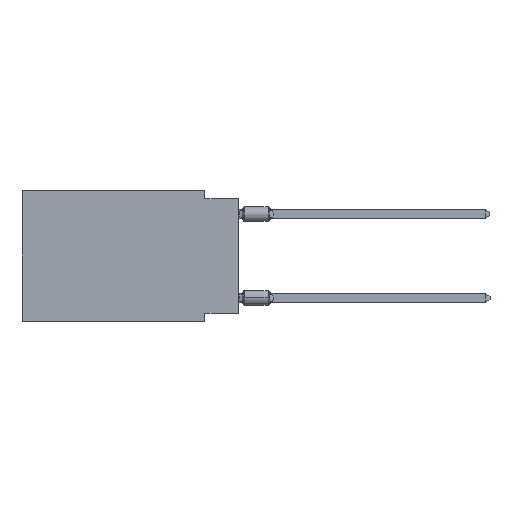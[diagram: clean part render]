
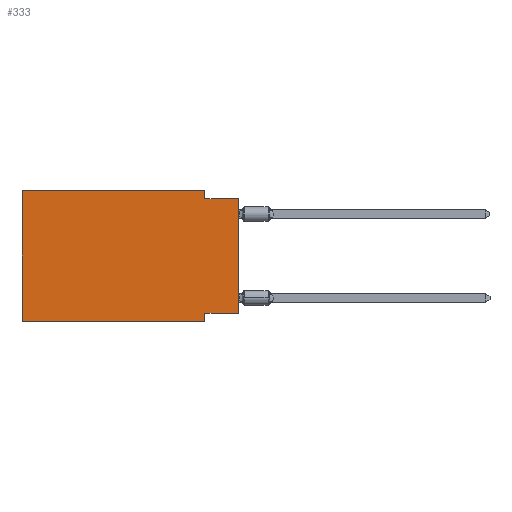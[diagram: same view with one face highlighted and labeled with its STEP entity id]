
A CAD part, left-side view. The second image highlights one B-rep face of the part: STEP entity #333.
In plain terms, the highlighted planar face has unit normal (-1, 0, 0).
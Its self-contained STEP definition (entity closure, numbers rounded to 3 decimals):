
#70 = ORIENTED_EDGE ( 'NONE', *, *, #18457, .F. ) ;
#333 = ADVANCED_FACE ( 'NONE', ( #9177 ), #6252, .F. ) ;
#515 = CARTESIAN_POINT ( 'NONE',  ( 0., 2.54, 0. ) ) ;
#806 = CARTESIAN_POINT ( 'NONE',  ( 0., 16.383, -9.906 ) ) ;
#1303 = CARTESIAN_POINT ( 'NONE',  ( 0., 16.383, 0. ) ) ;
#1512 = LINE ( 'NONE', #1303, #6906 ) ;
#1819 = DIRECTION ( 'NONE',  ( 0., 1., 0. ) ) ;
#1881 = ORIENTED_EDGE ( 'NONE', *, *, #11568, .T. ) ;
#2464 = CARTESIAN_POINT ( 'NONE',  ( 0., 2.54, -9.906 ) ) ;
#2805 = CARTESIAN_POINT ( 'NONE',  ( 0., 16.383, 0. ) ) ;
#3249 = LINE ( 'NONE', #7717, #7595 ) ;
#3280 = CARTESIAN_POINT ( 'NONE',  ( 0., 0., -0.635 ) ) ;
#3322 = CARTESIAN_POINT ( 'NONE',  ( 0., 16.383, -9.906 ) ) ;
#3542 = DIRECTION ( 'NONE',  ( 0., 0., 1. ) ) ;
#3617 = VECTOR ( 'NONE', #18863, 1000. ) ;
#4082 = EDGE_LOOP ( 'NONE', ( #5079, #5951, #11713, #5250, #19379, #1881, #17401, #70 ) ) ;
#4612 = CARTESIAN_POINT ( 'NONE',  ( 0., 2.54, -9.906 ) ) ;
#4690 = DIRECTION ( 'NONE',  ( 0., 0., 1. ) ) ;
#4871 = CARTESIAN_POINT ( 'NONE',  ( 0., 0., -9.271 ) ) ;
#5037 = VECTOR ( 'NONE', #3542, 1000. ) ;
#5079 = ORIENTED_EDGE ( 'NONE', *, *, #19835, .T. ) ;
#5250 = ORIENTED_EDGE ( 'NONE', *, *, #18360, .F. ) ;
#5699 = VERTEX_POINT ( 'NONE', #3280 ) ;
#5902 = VECTOR ( 'NONE', #11230, 1000. ) ;
#5951 = ORIENTED_EDGE ( 'NONE', *, *, #15155, .F. ) ;
#6066 = AXIS2_PLACEMENT_3D ( 'NONE', #2805, #7570, #9383 ) ;
#6252 = PLANE ( 'NONE',  #6066 ) ;
#6906 = VECTOR ( 'NONE', #10515, 1000. ) ;
#7210 = VECTOR ( 'NONE', #1819, 1000. ) ;
#7321 = LINE ( 'NONE', #2464, #13704 ) ;
#7570 = DIRECTION ( 'NONE',  ( 1., 0., 0. ) ) ;
#7595 = VECTOR ( 'NONE', #4690, 1000. ) ;
#7717 = CARTESIAN_POINT ( 'NONE',  ( 0., 16.383, 0. ) ) ;
#7720 = VERTEX_POINT ( 'NONE', #17162 ) ;
#9177 = FACE_OUTER_BOUND ( 'NONE', #4082, .T. ) ;
#9383 = DIRECTION ( 'NONE',  ( 0., 0., -1. ) ) ;
#9501 = DIRECTION ( 'NONE',  ( 0., -1., 0. ) ) ;
#10515 = DIRECTION ( 'NONE',  ( 0., -1., 0. ) ) ;
#11221 = CARTESIAN_POINT ( 'NONE',  ( 0., 2.54, -0.635 ) ) ;
#11230 = DIRECTION ( 'NONE',  ( 0., 0., -1. ) ) ;
#11568 = EDGE_CURVE ( 'NONE', #18259, #17651, #17174, .T. ) ;
#11713 = ORIENTED_EDGE ( 'NONE', *, *, #15934, .F. ) ;
#12145 = DIRECTION ( 'NONE',  ( 0., 0., -1. ) ) ;
#12157 = EDGE_CURVE ( 'NONE', #18259, #18945, #3249, .T. ) ;
#12621 = VERTEX_POINT ( 'NONE', #17177 ) ;
#12899 = CARTESIAN_POINT ( 'NONE',  ( 0., 0., -0.635 ) ) ;
#13018 = VERTEX_POINT ( 'NONE', #18285 ) ;
#13704 = VECTOR ( 'NONE', #12145, 1000. ) ;
#14364 = LINE ( 'NONE', #4871, #7210 ) ;
#15155 = EDGE_CURVE ( 'NONE', #19764, #5699, #15727, .T. ) ;
#15631 = VECTOR ( 'NONE', #9501, 1000. ) ;
#15727 = LINE ( 'NONE', #12899, #3617 ) ;
#15869 = LINE ( 'NONE', #515, #5902 ) ;
#15934 = EDGE_CURVE ( 'NONE', #13018, #19764, #15869, .T. ) ;
#17162 = CARTESIAN_POINT ( 'NONE',  ( 0., 0., -9.271 ) ) ;
#17174 = LINE ( 'NONE', #3322, #15631 ) ;
#17177 = CARTESIAN_POINT ( 'NONE',  ( 0., 2.54, -9.271 ) ) ;
#17384 = CARTESIAN_POINT ( 'NONE',  ( 0., 0., 0. ) ) ;
#17401 = ORIENTED_EDGE ( 'NONE', *, *, #19201, .F. ) ;
#17651 = VERTEX_POINT ( 'NONE', #4612 ) ;
#18259 = VERTEX_POINT ( 'NONE', #806 ) ;
#18285 = CARTESIAN_POINT ( 'NONE',  ( 0., 2.54, 0. ) ) ;
#18360 = EDGE_CURVE ( 'NONE', #18945, #13018, #1512, .T. ) ;
#18457 = EDGE_CURVE ( 'NONE', #7720, #12621, #14364, .T. ) ;
#18863 = DIRECTION ( 'NONE',  ( 0., -1., 0. ) ) ;
#18900 = LINE ( 'NONE', #17384, #5037 ) ;
#18945 = VERTEX_POINT ( 'NONE', #19225 ) ;
#19201 = EDGE_CURVE ( 'NONE', #12621, #17651, #7321, .T. ) ;
#19225 = CARTESIAN_POINT ( 'NONE',  ( 0., 16.383, 0. ) ) ;
#19379 = ORIENTED_EDGE ( 'NONE', *, *, #12157, .F. ) ;
#19764 = VERTEX_POINT ( 'NONE', #11221 ) ;
#19835 = EDGE_CURVE ( 'NONE', #7720, #5699, #18900, .T. ) ;
